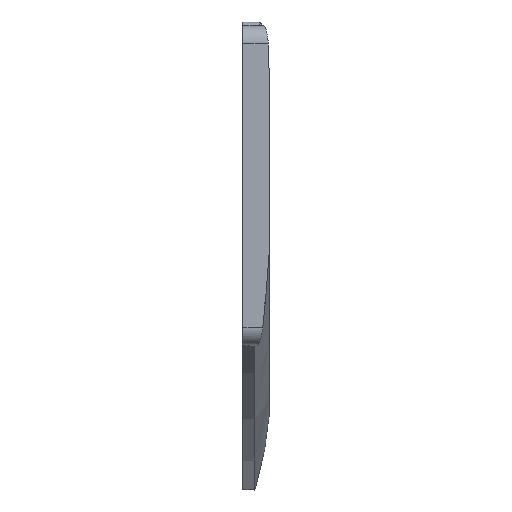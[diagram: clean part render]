
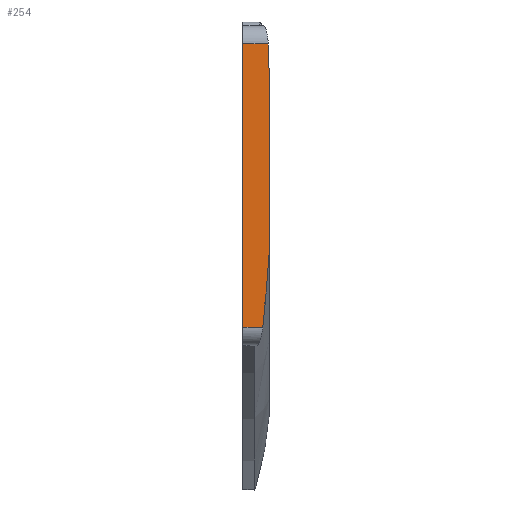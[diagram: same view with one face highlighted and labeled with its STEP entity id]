
A CAD part, top view. The second image highlights one B-rep face of the part: STEP entity #254.
In plain terms, the highlighted planar face has unit normal (0, 0, 1).
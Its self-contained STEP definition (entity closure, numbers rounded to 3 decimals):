
#93 = CARTESIAN_POINT ( 'NONE',  ( 8.1, -76.374, -2.355 ) ) ;
#110 = EDGE_CURVE ( 'NONE', #1363, #303, #996, .T. ) ;
#134 = CARTESIAN_POINT ( 'NONE',  ( 12.1, -81.012, -2.355 ) ) ;
#179 = VECTOR ( 'NONE', #1576, 1000. ) ;
#238 = CARTESIAN_POINT ( 'NONE',  ( 8.1, -76.374, -2.355 ) ) ;
#254 = ADVANCED_FACE ( 'NONE', ( #951 ), #1535, .F. ) ;
#258 = CARTESIAN_POINT ( 'NONE',  ( 12.051, -78., -2.355 ) ) ;
#262 = B_SPLINE_CURVE_WITH_KNOTS ( 'NONE', 3,
 ( #523, #1061, #1832, #1109 ),
 .UNSPECIFIED., .F., .F.,
 ( 4, 4 ),
 ( 0., 0.004 ),
 .UNSPECIFIED. ) ;
#277 = ORIENTED_EDGE ( 'NONE', *, *, #1513, .T. ) ;
#303 = VERTEX_POINT ( 'NONE', #859 ) ;
#316 = DIRECTION ( 'NONE',  ( -1., 0., 0. ) ) ;
#317 = CARTESIAN_POINT ( 'NONE',  ( 11.969, -110.335, -2.355 ) ) ;
#414 = ORIENTED_EDGE ( 'NONE', *, *, #1526, .F. ) ;
#450 = CARTESIAN_POINT ( 'NONE',  ( 12.1, -76.374, -2.355 ) ) ;
#461 = CARTESIAN_POINT ( 'NONE',  ( 12.1, -119.258, -2.355 ) ) ;
#479 = VECTOR ( 'NONE', #1674, 1000. ) ;
#508 = CARTESIAN_POINT ( 'NONE',  ( 12.1, -107.925, -2.355 ) ) ;
#513 = AXIS2_PLACEMENT_3D ( 'NONE', #984, #1527, #1687 ) ;
#523 = CARTESIAN_POINT ( 'NONE',  ( 11.122, -119.258, -2.355 ) ) ;
#568 = ORIENTED_EDGE ( 'NONE', *, *, #1285, .T. ) ;
#590 = EDGE_LOOP ( 'NONE', ( #817, #1236, #277, #1026, #414, #568, #1741 ) ) ;
#692 = CARTESIAN_POINT ( 'NONE',  ( 11.122, -119.258, -2.355 ) ) ;
#696 = VECTOR ( 'NONE', #316, 1000. ) ;
#705 = CARTESIAN_POINT ( 'NONE',  ( 12.1, -79.546, -2.355 ) ) ;
#814 = EDGE_CURVE ( 'NONE', #1242, #303, #909, .T. ) ;
#817 = ORIENTED_EDGE ( 'NONE', *, *, #814, .F. ) ;
#859 = CARTESIAN_POINT ( 'NONE',  ( 12.1, -107.925, -2.355 ) ) ;
#863 = CARTESIAN_POINT ( 'NONE',  ( 11.538, -115.142, -2.355 ) ) ;
#889 = EDGE_CURVE ( 'NONE', #1252, #1039, #1530, .T. ) ;
#909 = LINE ( 'NONE', #1382, #1292 ) ;
#951 = FACE_OUTER_BOUND ( 'NONE', #590, .T. ) ;
#984 = CARTESIAN_POINT ( 'NONE',  ( 12.1, -76.374, -2.355 ) ) ;
#996 = B_SPLINE_CURVE_WITH_KNOTS ( 'NONE', 3,
 ( #1657, #1801, #317, #508 ),
 .UNSPECIFIED., .F., .F.,
 ( 4, 4 ),
 ( 0., 0.007 ),
 .UNSPECIFIED. ) ;
#1008 = LINE ( 'NONE', #461, #179 ) ;
#1026 = ORIENTED_EDGE ( 'NONE', *, *, #889, .T. ) ;
#1039 = VERTEX_POINT ( 'NONE', #1701 ) ;
#1061 = CARTESIAN_POINT ( 'NONE',  ( 11.277, -117.888, -2.355 ) ) ;
#1102 = CARTESIAN_POINT ( 'NONE',  ( 12.1, -81.012, -2.355 ) ) ;
#1109 = CARTESIAN_POINT ( 'NONE',  ( 11.538, -115.142, -2.355 ) ) ;
#1148 = LINE ( 'NONE', #450, #696 ) ;
#1223 = VERTEX_POINT ( 'NONE', #1332 ) ;
#1236 = ORIENTED_EDGE ( 'NONE', *, *, #1401, .T. ) ;
#1242 = VERTEX_POINT ( 'NONE', #1102 ) ;
#1252 = VERTEX_POINT ( 'NONE', #93 ) ;
#1285 = EDGE_CURVE ( 'NONE', #1673, #1363, #262, .T. ) ;
#1292 = VECTOR ( 'NONE', #1794, 1000. ) ;
#1332 = CARTESIAN_POINT ( 'NONE',  ( 11.953, -76.374, -2.355 ) ) ;
#1363 = VERTEX_POINT ( 'NONE', #863 ) ;
#1382 = CARTESIAN_POINT ( 'NONE',  ( 12.1, -76.374, -2.355 ) ) ;
#1401 = EDGE_CURVE ( 'NONE', #1242, #1223, #1720, .T. ) ;
#1513 = EDGE_CURVE ( 'NONE', #1223, #1252, #1148, .T. ) ;
#1526 = EDGE_CURVE ( 'NONE', #1673, #1039, #1008, .T. ) ;
#1527 = DIRECTION ( 'NONE',  ( 0., 0., -1. ) ) ;
#1530 = LINE ( 'NONE', #238, #479 ) ;
#1535 = PLANE ( 'NONE',  #513 ) ;
#1576 = DIRECTION ( 'NONE',  ( -1., 0., 0. ) ) ;
#1657 = CARTESIAN_POINT ( 'NONE',  ( 11.538, -115.142, -2.355 ) ) ;
#1673 = VERTEX_POINT ( 'NONE', #692 ) ;
#1674 = DIRECTION ( 'NONE',  ( 0., -1., 0. ) ) ;
#1687 = DIRECTION ( 'NONE',  ( -1., 0., 0. ) ) ;
#1701 = CARTESIAN_POINT ( 'NONE',  ( 8.1, -119.258, -2.355 ) ) ;
#1720 = B_SPLINE_CURVE_WITH_KNOTS ( 'NONE', 3,
 ( #134, #705, #258, #1863 ),
 .UNSPECIFIED., .F., .F.,
 ( 4, 4 ),
 ( 0., 1. ),
 .UNSPECIFIED. ) ;
#1741 = ORIENTED_EDGE ( 'NONE', *, *, #110, .T. ) ;
#1794 = DIRECTION ( 'NONE',  ( 0., -1., 0. ) ) ;
#1801 = CARTESIAN_POINT ( 'NONE',  ( 11.769, -112.74, -2.355 ) ) ;
#1832 = CARTESIAN_POINT ( 'NONE',  ( 11.416, -116.516, -2.355 ) ) ;
#1863 = CARTESIAN_POINT ( 'NONE',  ( 11.953, -76.374, -2.355 ) ) ;
